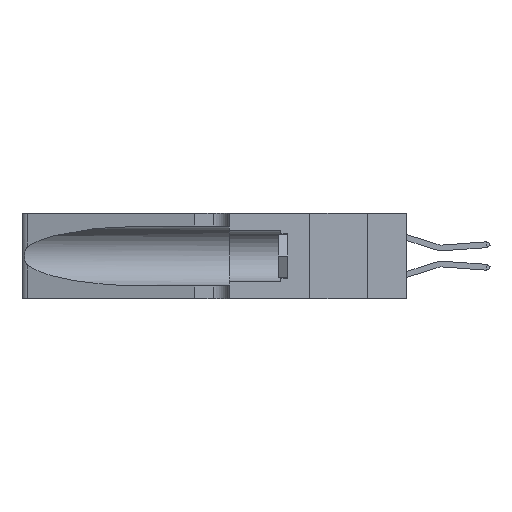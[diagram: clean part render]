
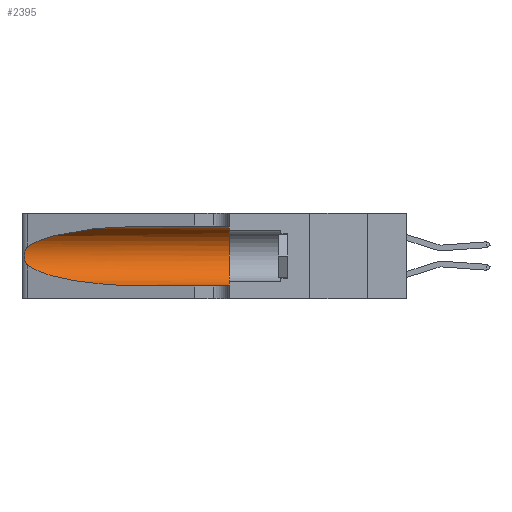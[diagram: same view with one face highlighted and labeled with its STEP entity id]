
A CAD part, left-side view. The second image highlights one B-rep face of the part: STEP entity #2395.
In plain terms, the highlighted cylindrical face has radius 3.308 mm (diameter 6.617 mm), a partial arc.
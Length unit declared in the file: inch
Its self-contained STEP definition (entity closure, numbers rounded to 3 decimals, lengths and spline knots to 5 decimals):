
#243 = VECTOR ( 'NONE', #19030, 39.37008 ) ;
#1242 = ORIENTED_EDGE ( 'NONE', *, *, #21756, .F. ) ;
#2395 = ADVANCED_FACE ( 'NONE', ( #12236 ), #18638, .F. ) ;
#2453 = AXIS2_PLACEMENT_3D ( 'NONE', #16162, #5264, #27053 ) ;
#2577 = CARTESIAN_POINT ( 'NONE',  ( 0.1305, 1.61858, 0.05475 ) ) ;
#2746 = CARTESIAN_POINT ( 'NONE',  ( 0.25789, 1.23486, 0.15765 ) ) ;
#3809 = EDGE_LOOP ( 'NONE', ( #24519, #33002, #12608, #7066, #1242, #17130 ) ) ;
#5264 = DIRECTION ( 'NONE',  ( 0., -1., 0. ) ) ;
#5566 = CARTESIAN_POINT ( 'NONE',  ( 0.25555, 1.22993, 0.14849 ) ) ;
#6153 = CARTESIAN_POINT ( 'NONE',  ( 0.1305, 0.72297, 0.31525 ) ) ;
#6871 = CARTESIAN_POINT ( 'NONE',  ( 0.1305, 0.72297, 0.05475 ) ) ;
#7066 = ORIENTED_EDGE ( 'NONE', *, *, #34317, .T. ) ;
#7205 =( BOUNDED_CURVE ( )  B_SPLINE_CURVE ( 3, ( #7604, #15771, #29355, #13147 ),
 .UNSPECIFIED., .F., .F. ) 
 B_SPLINE_CURVE_WITH_KNOTS ( ( 4, 4 ),
 ( 1.5708, 2.84003 ),
 .UNSPECIFIED. ) 
 CURVE ( )  GEOMETRIC_REPRESENTATION_ITEM ( )  RATIONAL_B_SPLINE_CURVE ( ( 1., 0.87, 0.87, 1. ) ) 
 REPRESENTATION_ITEM ( '' )  );
#7270 = VERTEX_POINT ( 'NONE', #23810 ) ;
#7604 = CARTESIAN_POINT ( 'NONE',  ( 0.1305, 0.72297, 0.31525 ) ) ;
#8036 = VERTEX_POINT ( 'NONE', #24031 ) ;
#9400 =( BOUNDED_CURVE ( )  B_SPLINE_CURVE ( 3, ( #33784, #14907, #23189, #6871 ),
 .UNSPECIFIED., .F., .T. ) 
 B_SPLINE_CURVE_WITH_KNOTS ( ( 4, 4 ),
 ( 3.44316, 4.71239 ),
 .UNSPECIFIED. ) 
 CURVE ( )  GEOMETRIC_REPRESENTATION_ITEM ( )  RATIONAL_B_SPLINE_CURVE ( ( 1., 0.87, 0.87, 1. ) ) 
 REPRESENTATION_ITEM ( '' )  );
#9951 = CIRCLE ( 'NONE', #30927, 0.13025 ) ;
#10834 = CARTESIAN_POINT ( 'NONE',  ( 0.25555, 1.22994, 0.2215 ) ) ;
#10950 = CARTESIAN_POINT ( 'NONE',  ( 0.25787, 1.23484, 0.2124 ) ) ;
#11353 = EDGE_CURVE ( 'NONE', #7270, #17079, #33707, .T. ) ;
#11702 = VECTOR ( 'NONE', #17194, 39.37008 ) ;
#12236 = FACE_OUTER_BOUND ( 'NONE', #3809, .T. ) ;
#12608 = ORIENTED_EDGE ( 'NONE', *, *, #33368, .T. ) ;
#13004 = DIRECTION ( 'NONE',  ( 0., 1., 0. ) ) ;
#13147 = CARTESIAN_POINT ( 'NONE',  ( 0.25487, 1.22718, 0.22369 ) ) ;
#13737 = CARTESIAN_POINT ( 'NONE',  ( 0.26018, 1.23835, 0.19895 ) ) ;
#13895 = CARTESIAN_POINT ( 'NONE',  ( 0.1305, 0.72297, 0.05475 ) ) ;
#13929 = VERTEX_POINT ( 'NONE', #13895 ) ;
#14434 = CARTESIAN_POINT ( 'NONE',  ( 0.1305, 1.61858, 0.31525 ) ) ;
#14907 = CARTESIAN_POINT ( 'NONE',  ( 0.2373, 1.15595, 0.08982 ) ) ;
#15771 = CARTESIAN_POINT ( 'NONE',  ( 0.18966, 0.96281, 0.31525 ) ) ;
#16162 = CARTESIAN_POINT ( 'NONE',  ( 0.1305, 1.61858, 0.185 ) ) ;
#16244 = CARTESIAN_POINT ( 'NONE',  ( 0.25487, 1.22718, 0.22369 ) ) ;
#16479 = CARTESIAN_POINT ( 'NONE',  ( 0.26075, 1.23896, 0.178 ) ) ;
#16831 = VERTEX_POINT ( 'NONE', #6153 ) ;
#17079 = VERTEX_POINT ( 'NONE', #18108 ) ;
#17130 = ORIENTED_EDGE ( 'NONE', *, *, #30764, .F. ) ;
#17194 = DIRECTION ( 'NONE',  ( 0., -1., 0. ) ) ;
#18108 = CARTESIAN_POINT ( 'NONE',  ( 0.25487, 1.22718, 0.14631 ) ) ;
#18638 = CYLINDRICAL_SURFACE ( 'NONE', #2453, 0.13025 ) ;
#19030 = DIRECTION ( 'NONE',  ( 0., -1., 0. ) ) ;
#19201 = CARTESIAN_POINT ( 'NONE',  ( 0.25856, 1.23593, 0.16098 ) ) ;
#21305 = EDGE_CURVE ( 'NONE', #16831, #7270, #7205, .T. ) ;
#21756 = EDGE_CURVE ( 'NONE', #28610, #8036, #9951, .T. ) ;
#21906 = CARTESIAN_POINT ( 'NONE',  ( 0.25639, 1.23186, 0.15144 ) ) ;
#22946 = CARTESIAN_POINT ( 'NONE',  ( 0.1305, 0.35, 0.31525 ) ) ;
#23189 = CARTESIAN_POINT ( 'NONE',  ( 0.18966, 0.96281, 0.05475 ) ) ;
#23810 = CARTESIAN_POINT ( 'NONE',  ( 0.25487, 1.22718, 0.22369 ) ) ;
#24031 = CARTESIAN_POINT ( 'NONE',  ( 0.1305, 0.35, 0.05475 ) ) ;
#24519 = ORIENTED_EDGE ( 'NONE', *, *, #21305, .T. ) ;
#24641 = CARTESIAN_POINT ( 'NONE',  ( 0.25487, 1.22718, 0.14631 ) ) ;
#27053 = DIRECTION ( 'NONE',  ( 0., 0., -1. ) ) ;
#27242 = CARTESIAN_POINT ( 'NONE',  ( 0.25639, 1.23184, 0.21858 ) ) ;
#28610 = VERTEX_POINT ( 'NONE', #22946 ) ;
#29205 = CARTESIAN_POINT ( 'NONE',  ( 0.1305, 0.35, 0.185 ) ) ;
#29355 = CARTESIAN_POINT ( 'NONE',  ( 0.2373, 1.15595, 0.28018 ) ) ;
#29389 = LINE ( 'NONE', #2577, #243 ) ;
#29925 = CARTESIAN_POINT ( 'NONE',  ( 0.25854, 1.2359, 0.20912 ) ) ;
#30764 = EDGE_CURVE ( 'NONE', #16831, #28610, #33287, .T. ) ;
#30927 = AXIS2_PLACEMENT_3D ( 'NONE', #29205, #13004, #31896 ) ;
#31896 = DIRECTION ( 'NONE',  ( 0., 0., 1. ) ) ;
#32620 = CARTESIAN_POINT ( 'NONE',  ( 0.26075, 1.23896, 0.19203 ) ) ;
#33002 = ORIENTED_EDGE ( 'NONE', *, *, #11353, .T. ) ;
#33287 = LINE ( 'NONE', #14434, #11702 ) ;
#33368 = EDGE_CURVE ( 'NONE', #17079, #13929, #9400, .T. ) ;
#33707 = B_SPLINE_CURVE_WITH_KNOTS ( 'NONE', 3,
 ( #16244, #10834, #27242, #10950, #29925, #13737, #32620, #16479, #35314, #19201, #2746, #21906, #5566, #24641 ),
 .UNSPECIFIED., .F., .F.,
 ( 4, 2, 2, 2, 2, 2, 4 ),
 ( 0., 0.00027, 0.00053, 0.00107, 0.0016, 0.00187, 0.00214 ),
 .UNSPECIFIED. ) ;
#33784 = CARTESIAN_POINT ( 'NONE',  ( 0.25487, 1.22718, 0.14631 ) ) ;
#34317 = EDGE_CURVE ( 'NONE', #13929, #8036, #29389, .T. ) ;
#35314 = CARTESIAN_POINT ( 'NONE',  ( 0.26017, 1.23833, 0.17102 ) ) ;
